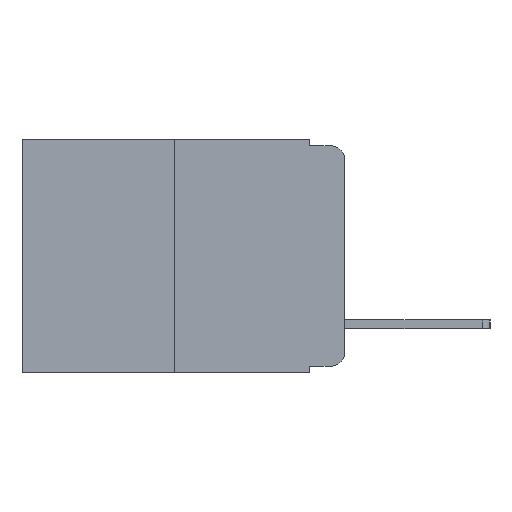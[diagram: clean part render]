
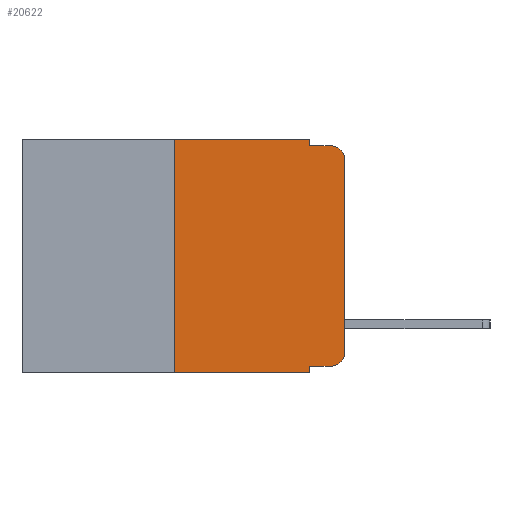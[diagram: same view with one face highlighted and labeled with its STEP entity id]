
A CAD part, left-side view. The second image highlights one B-rep face of the part: STEP entity #20622.
In plain terms, the highlighted planar face has unit normal (-1, 0, 0).
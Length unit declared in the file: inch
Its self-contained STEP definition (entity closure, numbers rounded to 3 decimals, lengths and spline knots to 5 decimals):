
#21 = VERTEX_POINT ( 'NONE', #14714 ) ;
#97 = LINE ( 'NONE', #16013, #16754 ) ;
#248 = ORIENTED_EDGE ( 'NONE', *, *, #2174, .T. ) ;
#1060 = EDGE_CURVE ( 'NONE', #18640, #15360, #10983, .T. ) ;
#1135 = DIRECTION ( 'NONE',  ( 0., -1., 0. ) ) ;
#1165 = DIRECTION ( 'NONE',  ( 0., 0., -1. ) ) ;
#2174 = EDGE_CURVE ( 'NONE', #5603, #18640, #19022, .T. ) ;
#2527 = LINE ( 'NONE', #8064, #18030 ) ;
#2626 = ORIENTED_EDGE ( 'NONE', *, *, #5782, .T. ) ;
#2894 = AXIS2_PLACEMENT_3D ( 'NONE', #4422, #10969, #1165 ) ;
#3166 = DIRECTION ( 'NONE',  ( 0., -1., 0. ) ) ;
#3170 = EDGE_LOOP ( 'NONE', ( #6804, #10714, #5133, #17733, #17944, #3803, #2626, #3189, #248, #8703 ) ) ;
#3189 = ORIENTED_EDGE ( 'NONE', *, *, #5480, .F. ) ;
#3604 = CARTESIAN_POINT ( 'NONE',  ( 0., 0.051, 0. ) ) ;
#3803 = ORIENTED_EDGE ( 'NONE', *, *, #6590, .F. ) ;
#3907 = LINE ( 'NONE', #17924, #8269 ) ;
#4265 = DIRECTION ( 'NONE',  ( 0., 0., 1. ) ) ;
#4422 = CARTESIAN_POINT ( 'NONE',  ( 0., 0.473, 0. ) ) ;
#4842 = DIRECTION ( 'NONE',  ( 0., 0., -1. ) ) ;
#5133 = ORIENTED_EDGE ( 'NONE', *, *, #9833, .F. ) ;
#5188 = DIRECTION ( 'NONE',  ( 0., -1., 0. ) ) ;
#5480 = EDGE_CURVE ( 'NONE', #5603, #14160, #19581, .T. ) ;
#5603 = VERTEX_POINT ( 'NONE', #8818 ) ;
#5782 = EDGE_CURVE ( 'NONE', #10351, #14160, #18374, .T. ) ;
#6088 = PLANE ( 'NONE',  #2894 ) ;
#6383 = CARTESIAN_POINT ( 'NONE',  ( 0., 0.02, -0.03 ) ) ;
#6520 = EDGE_CURVE ( 'NONE', #8930, #9440, #2527, .T. ) ;
#6590 = EDGE_CURVE ( 'NONE', #10351, #8930, #9664, .T. ) ;
#6804 = ORIENTED_EDGE ( 'NONE', *, *, #13022, .T. ) ;
#6867 = DIRECTION ( 'NONE',  ( 0., -1., 0. ) ) ;
#6992 = VECTOR ( 'NONE', #13336, 39.37008 ) ;
#7149 = VECTOR ( 'NONE', #4265, 39.37008 ) ;
#7711 = EDGE_CURVE ( 'NONE', #9440, #14364, #97, .T. ) ;
#7981 = CIRCLE ( 'NONE', #19072, 0.02 ) ;
#8036 = DIRECTION ( 'NONE',  ( 0., 0., -1. ) ) ;
#8064 = CARTESIAN_POINT ( 'NONE',  ( 0., 0.473, 0. ) ) ;
#8196 = DIRECTION ( 'NONE',  ( 0., 0., 1. ) ) ;
#8269 = VECTOR ( 'NONE', #6867, 39.37008 ) ;
#8703 = ORIENTED_EDGE ( 'NONE', *, *, #1060, .T. ) ;
#8818 = CARTESIAN_POINT ( 'NONE',  ( 0., 0.051, -0.333 ) ) ;
#8930 = VERTEX_POINT ( 'NONE', #10713 ) ;
#9440 = VERTEX_POINT ( 'NONE', #16623 ) ;
#9664 = LINE ( 'NONE', #20739, #17057 ) ;
#9833 = EDGE_CURVE ( 'NONE', #14364, #18997, #3907, .T. ) ;
#10000 = VECTOR ( 'NONE', #1135, 39.37008 ) ;
#10351 = VERTEX_POINT ( 'NONE', #20730 ) ;
#10686 = VECTOR ( 'NONE', #5188, 39.37008 ) ;
#10713 = CARTESIAN_POINT ( 'NONE',  ( 0., 0.25, 0. ) ) ;
#10714 = ORIENTED_EDGE ( 'NONE', *, *, #10928, .T. ) ;
#10928 = EDGE_CURVE ( 'NONE', #21, #18997, #7981, .T. ) ;
#10969 = DIRECTION ( 'NONE',  ( 1., 0., 0. ) ) ;
#10983 = CIRCLE ( 'NONE', #18689, 0.02 ) ;
#11081 = FACE_OUTER_BOUND ( 'NONE', #3170, .T. ) ;
#12262 = CARTESIAN_POINT ( 'NONE',  ( 0., 0., -0.313 ) ) ;
#12462 = CARTESIAN_POINT ( 'NONE',  ( 0., 0.02, -0.01 ) ) ;
#13022 = EDGE_CURVE ( 'NONE', #15360, #21, #19719, .T. ) ;
#13336 = DIRECTION ( 'NONE',  ( 0., 0., -1. ) ) ;
#14160 = VERTEX_POINT ( 'NONE', #19777 ) ;
#14364 = VERTEX_POINT ( 'NONE', #15956 ) ;
#14714 = CARTESIAN_POINT ( 'NONE',  ( 0., 0., -0.03 ) ) ;
#15360 = VERTEX_POINT ( 'NONE', #12262 ) ;
#15956 = CARTESIAN_POINT ( 'NONE',  ( 0., 0.051, -0.01 ) ) ;
#16013 = CARTESIAN_POINT ( 'NONE',  ( 0., 0.051, 0. ) ) ;
#16623 = CARTESIAN_POINT ( 'NONE',  ( 0., 0.051, 0. ) ) ;
#16754 = VECTOR ( 'NONE', #4842, 39.37008 ) ;
#16915 = CARTESIAN_POINT ( 'NONE',  ( 0., 0.02, -0.333 ) ) ;
#16977 = CARTESIAN_POINT ( 'NONE',  ( 0., 0., 0. ) ) ;
#17057 = VECTOR ( 'NONE', #8196, 39.37008 ) ;
#17463 = DIRECTION ( 'NONE',  ( -1., 0., 0. ) ) ;
#17733 = ORIENTED_EDGE ( 'NONE', *, *, #7711, .F. ) ;
#17924 = CARTESIAN_POINT ( 'NONE',  ( 0., 0.051, -0.01 ) ) ;
#17944 = ORIENTED_EDGE ( 'NONE', *, *, #6520, .F. ) ;
#18030 = VECTOR ( 'NONE', #3166, 39.37008 ) ;
#18374 = LINE ( 'NONE', #20280, #10000 ) ;
#18507 = DIRECTION ( 'NONE',  ( -1., 0., 0. ) ) ;
#18558 = CARTESIAN_POINT ( 'NONE',  ( 0., 0.02, -0.313 ) ) ;
#18640 = VERTEX_POINT ( 'NONE', #16915 ) ;
#18689 = AXIS2_PLACEMENT_3D ( 'NONE', #18558, #18507, #19293 ) ;
#18997 = VERTEX_POINT ( 'NONE', #12462 ) ;
#19022 = LINE ( 'NONE', #19494, #10686 ) ;
#19072 = AXIS2_PLACEMENT_3D ( 'NONE', #6383, #17463, #8036 ) ;
#19293 = DIRECTION ( 'NONE',  ( 0., 0., -1. ) ) ;
#19494 = CARTESIAN_POINT ( 'NONE',  ( 0., 0.051, -0.333 ) ) ;
#19581 = LINE ( 'NONE', #3604, #6992 ) ;
#19719 = LINE ( 'NONE', #16977, #7149 ) ;
#19777 = CARTESIAN_POINT ( 'NONE',  ( 0., 0.051, -0.343 ) ) ;
#20280 = CARTESIAN_POINT ( 'NONE',  ( 0., 0.473, -0.343 ) ) ;
#20622 = ADVANCED_FACE ( 'NONE', ( #11081 ), #6088, .F. ) ;
#20730 = CARTESIAN_POINT ( 'NONE',  ( 0., 0.25, -0.343 ) ) ;
#20739 = CARTESIAN_POINT ( 'NONE',  ( 0., 0.25, 0. ) ) ;
